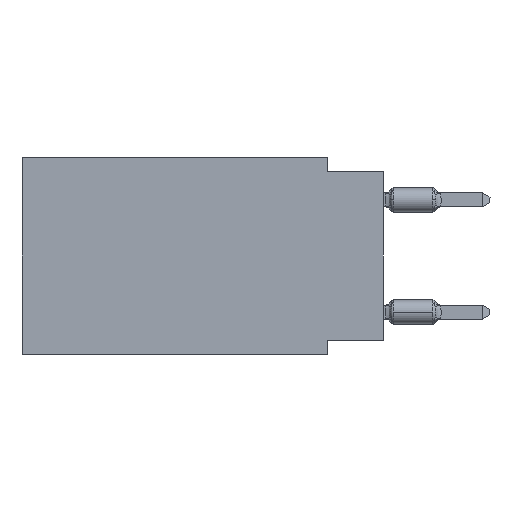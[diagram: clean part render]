
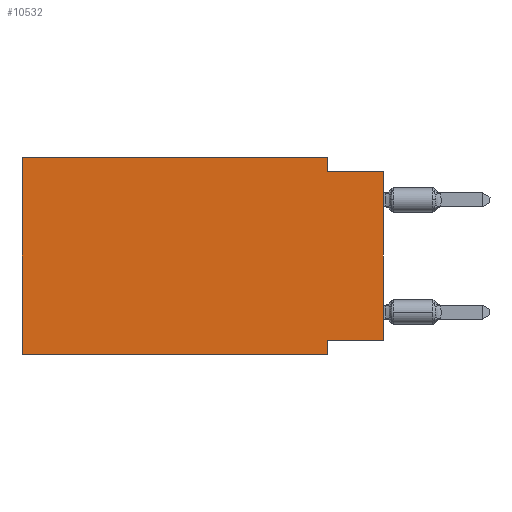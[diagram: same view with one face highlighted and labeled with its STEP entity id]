
A CAD part, left-side view. The second image highlights one B-rep face of the part: STEP entity #10532.
In plain terms, the highlighted planar face has unit normal (-1, 0, 0).
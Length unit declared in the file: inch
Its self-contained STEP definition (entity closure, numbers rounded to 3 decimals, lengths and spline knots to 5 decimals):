
#135 = AXIS2_PLACEMENT_3D ( 'NONE', #7292, #7940, #2631 ) ;
#145 = VECTOR ( 'NONE', #241, 39.37008 ) ;
#241 = DIRECTION ( 'NONE',  ( 0., -1., 0. ) ) ;
#259 = VERTEX_POINT ( 'NONE', #1910 ) ;
#268 = VERTEX_POINT ( 'NONE', #8066 ) ;
#858 = CARTESIAN_POINT ( 'NONE',  ( 0., 0., -0.025 ) ) ;
#1160 = LINE ( 'NONE', #4152, #6208 ) ;
#1188 = VECTOR ( 'NONE', #7727, 39.37008 ) ;
#1481 = CARTESIAN_POINT ( 'NONE',  ( 0., 0.1, -0.35 ) ) ;
#1724 = LINE ( 'NONE', #4974, #4450 ) ;
#1789 = DIRECTION ( 'NONE',  ( 0., 0., -1. ) ) ;
#1834 = ORIENTED_EDGE ( 'NONE', *, *, #8201, .F. ) ;
#1910 = CARTESIAN_POINT ( 'NONE',  ( 0., 0.645, -0.35 ) ) ;
#1960 = VERTEX_POINT ( 'NONE', #11952 ) ;
#2166 = EDGE_CURVE ( 'NONE', #1960, #12335, #4212, .T. ) ;
#2631 = DIRECTION ( 'NONE',  ( 0., 0., -1. ) ) ;
#2829 = CARTESIAN_POINT ( 'NONE',  ( 0., 0.645, 0. ) ) ;
#3036 = DIRECTION ( 'NONE',  ( 0., 0., -1. ) ) ;
#3109 = DIRECTION ( 'NONE',  ( 0., 0., 1. ) ) ;
#3358 = CARTESIAN_POINT ( 'NONE',  ( 0., 0., -0.025 ) ) ;
#3524 = LINE ( 'NONE', #6963, #1188 ) ;
#3745 = FACE_OUTER_BOUND ( 'NONE', #8320, .T. ) ;
#4072 = EDGE_CURVE ( 'NONE', #259, #268, #5211, .T. ) ;
#4152 = CARTESIAN_POINT ( 'NONE',  ( 0., 0., 0. ) ) ;
#4212 = LINE ( 'NONE', #7368, #10581 ) ;
#4450 = VECTOR ( 'NONE', #1789, 39.37008 ) ;
#4910 = EDGE_CURVE ( 'NONE', #12694, #10095, #11788, .T. ) ;
#4974 = CARTESIAN_POINT ( 'NONE',  ( 0., 0.1, 0. ) ) ;
#5080 = DIRECTION ( 'NONE',  ( 0., 0., 1. ) ) ;
#5211 = LINE ( 'NONE', #7269, #12717 ) ;
#5481 = EDGE_CURVE ( 'NONE', #13347, #12694, #1724, .T. ) ;
#5499 = EDGE_CURVE ( 'NONE', #7125, #10095, #1160, .T. ) ;
#6208 = VECTOR ( 'NONE', #3109, 39.37008 ) ;
#6819 = LINE ( 'NONE', #7848, #10018 ) ;
#6963 = CARTESIAN_POINT ( 'NONE',  ( 0., 0., -0.325 ) ) ;
#7125 = VERTEX_POINT ( 'NONE', #12684 ) ;
#7269 = CARTESIAN_POINT ( 'NONE',  ( 0., 0.645, 0. ) ) ;
#7292 = CARTESIAN_POINT ( 'NONE',  ( 0., 0.645, 0. ) ) ;
#7325 = ORIENTED_EDGE ( 'NONE', *, *, #4072, .F. ) ;
#7368 = CARTESIAN_POINT ( 'NONE',  ( 0., 0.1, -0.35 ) ) ;
#7623 = VECTOR ( 'NONE', #12552, 39.37008 ) ;
#7727 = DIRECTION ( 'NONE',  ( 0., 1., 0. ) ) ;
#7848 = CARTESIAN_POINT ( 'NONE',  ( 0., 0.645, -0.35 ) ) ;
#7940 = DIRECTION ( 'NONE',  ( 1., 0., 0. ) ) ;
#8026 = ORIENTED_EDGE ( 'NONE', *, *, #2166, .F. ) ;
#8066 = CARTESIAN_POINT ( 'NONE',  ( 0., 0.645, 0. ) ) ;
#8201 = EDGE_CURVE ( 'NONE', #7125, #1960, #3524, .T. ) ;
#8219 = CARTESIAN_POINT ( 'NONE',  ( 0., 0.1, 0. ) ) ;
#8320 = EDGE_LOOP ( 'NONE', ( #10415, #11218, #12438, #10016, #7325, #9779, #8026, #1834 ) ) ;
#9262 = EDGE_CURVE ( 'NONE', #259, #12335, #6819, .T. ) ;
#9779 = ORIENTED_EDGE ( 'NONE', *, *, #9262, .T. ) ;
#10016 = ORIENTED_EDGE ( 'NONE', *, *, #12498, .F. ) ;
#10018 = VECTOR ( 'NONE', #11047, 39.37008 ) ;
#10095 = VERTEX_POINT ( 'NONE', #858 ) ;
#10415 = ORIENTED_EDGE ( 'NONE', *, *, #5499, .T. ) ;
#10532 = ADVANCED_FACE ( 'NONE', ( #3745 ), #12103, .F. ) ;
#10581 = VECTOR ( 'NONE', #3036, 39.37008 ) ;
#11047 = DIRECTION ( 'NONE',  ( 0., -1., 0. ) ) ;
#11218 = ORIENTED_EDGE ( 'NONE', *, *, #4910, .F. ) ;
#11788 = LINE ( 'NONE', #3358, #145 ) ;
#11793 = CARTESIAN_POINT ( 'NONE',  ( 0., 0.1, -0.025 ) ) ;
#11952 = CARTESIAN_POINT ( 'NONE',  ( 0., 0.1, -0.325 ) ) ;
#12103 = PLANE ( 'NONE',  #135 ) ;
#12286 = LINE ( 'NONE', #2829, #7623 ) ;
#12335 = VERTEX_POINT ( 'NONE', #1481 ) ;
#12438 = ORIENTED_EDGE ( 'NONE', *, *, #5481, .F. ) ;
#12498 = EDGE_CURVE ( 'NONE', #268, #13347, #12286, .T. ) ;
#12552 = DIRECTION ( 'NONE',  ( 0., -1., 0. ) ) ;
#12684 = CARTESIAN_POINT ( 'NONE',  ( 0., 0., -0.325 ) ) ;
#12694 = VERTEX_POINT ( 'NONE', #11793 ) ;
#12717 = VECTOR ( 'NONE', #5080, 39.37008 ) ;
#13347 = VERTEX_POINT ( 'NONE', #8219 ) ;
